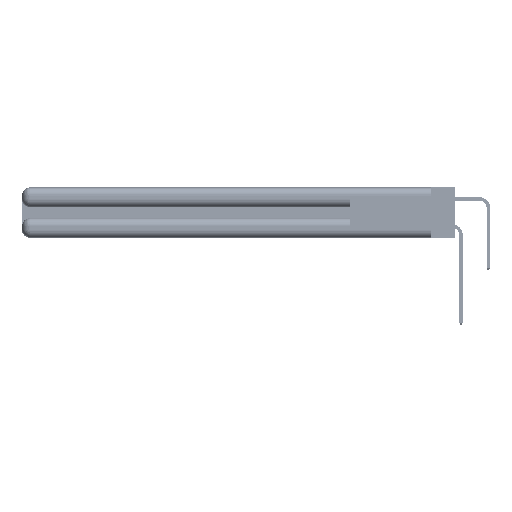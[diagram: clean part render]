
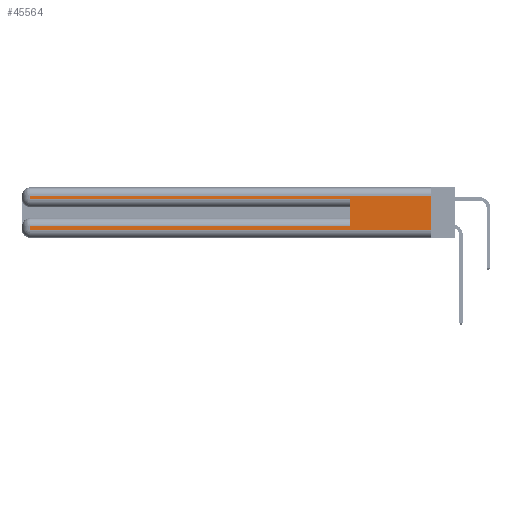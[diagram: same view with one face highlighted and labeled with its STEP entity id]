
A CAD part, left-side view. The second image highlights one B-rep face of the part: STEP entity #45564.
In plain terms, the highlighted planar face has unit normal (-1, 0, 0).
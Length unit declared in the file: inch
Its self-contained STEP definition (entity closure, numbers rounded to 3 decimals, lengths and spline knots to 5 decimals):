
#897 = ORIENTED_EDGE ( 'NONE', *, *, #48845, .T. ) ;
#2615 = LINE ( 'NONE', #27241, #15662 ) ;
#2770 = EDGE_CURVE ( 'NONE', #28497, #42533, #2615, .T. ) ;
#5426 = EDGE_LOOP ( 'NONE', ( #13464, #34359, #897, #49632, #35004, #6754, #45393, #7250 ) ) ;
#5675 = VERTEX_POINT ( 'NONE', #40887 ) ;
#5989 = LINE ( 'NONE', #17320, #50903 ) ;
#6734 = EDGE_CURVE ( 'NONE', #5675, #28497, #39631, .T. ) ;
#6754 = ORIENTED_EDGE ( 'NONE', *, *, #6734, .T. ) ;
#7250 = ORIENTED_EDGE ( 'NONE', *, *, #10278, .T. ) ;
#10102 = VERTEX_POINT ( 'NONE', #44502 ) ;
#10278 = EDGE_CURVE ( 'NONE', #42533, #10102, #27524, .T. ) ;
#11027 = DIRECTION ( 'NONE',  ( 0., 0., -1. ) ) ;
#13292 = DIRECTION ( 'NONE',  ( 0., 0., 1. ) ) ;
#13464 = ORIENTED_EDGE ( 'NONE', *, *, #41772, .F. ) ;
#13638 = CARTESIAN_POINT ( 'NONE',  ( 0., 0.6, 0.285 ) ) ;
#15065 = CARTESIAN_POINT ( 'NONE',  ( 0., 0., 0.085 ) ) ;
#15662 = VECTOR ( 'NONE', #11027, 39.37008 ) ;
#17211 = CARTESIAN_POINT ( 'NONE',  ( 0., 0., 0.06 ) ) ;
#17320 = CARTESIAN_POINT ( 'NONE',  ( 0., 0.6, 0.145 ) ) ;
#17763 = EDGE_CURVE ( 'NONE', #22939, #47167, #39773, .T. ) ;
#19305 = LINE ( 'NONE', #34412, #46790 ) ;
#22656 = EDGE_CURVE ( 'NONE', #5675, #46735, #5989, .T. ) ;
#22939 = VERTEX_POINT ( 'NONE', #31073 ) ;
#23070 = CARTESIAN_POINT ( 'NONE',  ( 0., 2.94, 0.285 ) ) ;
#23733 = VECTOR ( 'NONE', #41574, 39.37008 ) ;
#24217 = AXIS2_PLACEMENT_3D ( 'NONE', #29490, #26311, #50059 ) ;
#26311 = DIRECTION ( 'NONE',  ( 1., 0., 0. ) ) ;
#27189 = CARTESIAN_POINT ( 'NONE',  ( 0., 2.94, 0.06 ) ) ;
#27241 = CARTESIAN_POINT ( 'NONE',  ( 0., 2.94, 0.37 ) ) ;
#27524 = LINE ( 'NONE', #17211, #23733 ) ;
#28497 = VERTEX_POINT ( 'NONE', #44995 ) ;
#29378 = EDGE_CURVE ( 'NONE', #46373, #46735, #40343, .T. ) ;
#29490 = CARTESIAN_POINT ( 'NONE',  ( 0., 0., 0.37 ) ) ;
#29793 = VECTOR ( 'NONE', #51439, 39.37008 ) ;
#30439 = CARTESIAN_POINT ( 'NONE',  ( 0., 2.94, 0.31 ) ) ;
#31073 = CARTESIAN_POINT ( 'NONE',  ( 0., 0., 0.31 ) ) ;
#33577 = DIRECTION ( 'NONE',  ( 0., 1., 0. ) ) ;
#34359 = ORIENTED_EDGE ( 'NONE', *, *, #17763, .T. ) ;
#34412 = CARTESIAN_POINT ( 'NONE',  ( 0., 0., 0.37 ) ) ;
#34805 = VECTOR ( 'NONE', #33577, 39.37008 ) ;
#35004 = ORIENTED_EDGE ( 'NONE', *, *, #22656, .F. ) ;
#39317 = CARTESIAN_POINT ( 'NONE',  ( 0., 2.94, 0.37 ) ) ;
#39631 = LINE ( 'NONE', #15065, #42120 ) ;
#39773 = LINE ( 'NONE', #41352, #34805 ) ;
#39837 = DIRECTION ( 'NONE',  ( 0., 0., -1. ) ) ;
#40343 = LINE ( 'NONE', #47432, #29793 ) ;
#40887 = CARTESIAN_POINT ( 'NONE',  ( 0., 0.6, 0.085 ) ) ;
#41352 = CARTESIAN_POINT ( 'NONE',  ( 0., 0., 0.31 ) ) ;
#41363 = FACE_OUTER_BOUND ( 'NONE', #5426, .T. ) ;
#41574 = DIRECTION ( 'NONE',  ( 0., -1., 0. ) ) ;
#41772 = EDGE_CURVE ( 'NONE', #22939, #10102, #19305, .T. ) ;
#42120 = VECTOR ( 'NONE', #42956, 39.37008 ) ;
#42207 = DIRECTION ( 'NONE',  ( 0., 0., -1. ) ) ;
#42533 = VERTEX_POINT ( 'NONE', #27189 ) ;
#42849 = VECTOR ( 'NONE', #39837, 39.37008 ) ;
#42956 = DIRECTION ( 'NONE',  ( 0., 1., 0. ) ) ;
#44502 = CARTESIAN_POINT ( 'NONE',  ( 0., 0., 0.06 ) ) ;
#44995 = CARTESIAN_POINT ( 'NONE',  ( 0., 2.94, 0.085 ) ) ;
#45393 = ORIENTED_EDGE ( 'NONE', *, *, #2770, .T. ) ;
#45564 = ADVANCED_FACE ( 'NONE', ( #41363 ), #49896, .F. ) ;
#46373 = VERTEX_POINT ( 'NONE', #23070 ) ;
#46646 = LINE ( 'NONE', #39317, #42849 ) ;
#46735 = VERTEX_POINT ( 'NONE', #13638 ) ;
#46790 = VECTOR ( 'NONE', #42207, 39.37008 ) ;
#47167 = VERTEX_POINT ( 'NONE', #30439 ) ;
#47432 = CARTESIAN_POINT ( 'NONE',  ( 0., 0., 0.285 ) ) ;
#48845 = EDGE_CURVE ( 'NONE', #47167, #46373, #46646, .T. ) ;
#49632 = ORIENTED_EDGE ( 'NONE', *, *, #29378, .T. ) ;
#49896 = PLANE ( 'NONE',  #24217 ) ;
#50059 = DIRECTION ( 'NONE',  ( 0., 0., -1. ) ) ;
#50903 = VECTOR ( 'NONE', #13292, 39.37008 ) ;
#51439 = DIRECTION ( 'NONE',  ( 0., -1., 0. ) ) ;
